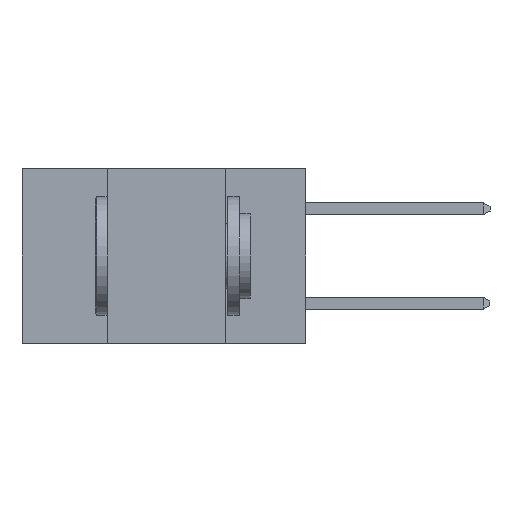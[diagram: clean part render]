
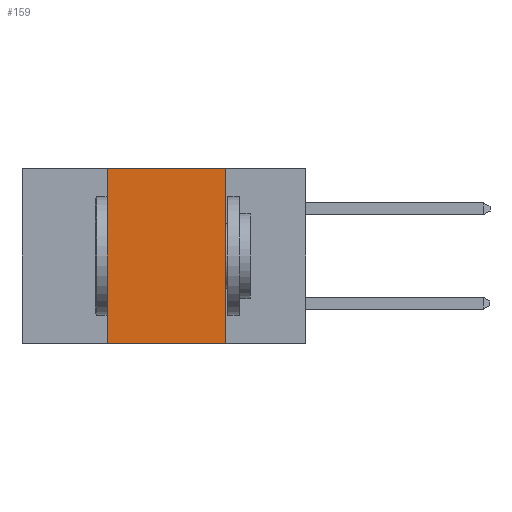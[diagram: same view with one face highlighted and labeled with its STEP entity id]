
A CAD part, left-side view. The second image highlights one B-rep face of the part: STEP entity #159.
In plain terms, the highlighted planar face has unit normal (-1, 0, 0).
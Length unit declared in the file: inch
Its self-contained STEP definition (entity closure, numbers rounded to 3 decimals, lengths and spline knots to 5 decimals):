
#159 = ADVANCED_FACE ( 'NONE', ( #12112 ), #9676, .F. ) ;
#357 = ORIENTED_EDGE ( 'NONE', *, *, #2655, .T. ) ;
#599 = CARTESIAN_POINT ( 'NONE',  ( 0., 0.17, -0.37 ) ) ;
#726 = VECTOR ( 'NONE', #13380, 39.37008 ) ;
#1174 = ORIENTED_EDGE ( 'NONE', *, *, #9477, .F. ) ;
#1383 = CARTESIAN_POINT ( 'NONE',  ( 0., 0.42, 0. ) ) ;
#2437 = DIRECTION ( 'NONE',  ( 0., -1., 0. ) ) ;
#2655 = EDGE_CURVE ( 'NONE', #13415, #5528, #12569, .T. ) ;
#3301 = VERTEX_POINT ( 'NONE', #3535 ) ;
#3443 = EDGE_CURVE ( 'NONE', #13415, #3873, #6007, .T. ) ;
#3535 = CARTESIAN_POINT ( 'NONE',  ( 0., 0.17, 0. ) ) ;
#3538 = LINE ( 'NONE', #6729, #726 ) ;
#3873 = VERTEX_POINT ( 'NONE', #7276 ) ;
#4242 = EDGE_CURVE ( 'NONE', #3301, #5528, #7829, .T. ) ;
#5293 = CARTESIAN_POINT ( 'NONE',  ( 0., 0.17, 0. ) ) ;
#5528 = VERTEX_POINT ( 'NONE', #599 ) ;
#5921 = ORIENTED_EDGE ( 'NONE', *, *, #3443, .F. ) ;
#6007 = LINE ( 'NONE', #1383, #8735 ) ;
#6057 = CARTESIAN_POINT ( 'NONE',  ( 0., 0.6, -0.37 ) ) ;
#6729 = CARTESIAN_POINT ( 'NONE',  ( 0., 0.6, 0. ) ) ;
#6868 = ORIENTED_EDGE ( 'NONE', *, *, #4242, .F. ) ;
#7229 = DIRECTION ( 'NONE',  ( 1., 0., 0. ) ) ;
#7276 = CARTESIAN_POINT ( 'NONE',  ( 0., 0.42, 0. ) ) ;
#7491 = CARTESIAN_POINT ( 'NONE',  ( 0., 0.6, 0. ) ) ;
#7829 = LINE ( 'NONE', #5293, #10468 ) ;
#8735 = VECTOR ( 'NONE', #11108, 39.37008 ) ;
#8996 = CARTESIAN_POINT ( 'NONE',  ( 0., 0.42, -0.37 ) ) ;
#9279 = DIRECTION ( 'NONE',  ( 0., 0., -1. ) ) ;
#9477 = EDGE_CURVE ( 'NONE', #3873, #3301, #3538, .T. ) ;
#9676 = PLANE ( 'NONE',  #14174 ) ;
#10207 = DIRECTION ( 'NONE',  ( 0., 0., -1. ) ) ;
#10468 = VECTOR ( 'NONE', #10207, 39.37008 ) ;
#11108 = DIRECTION ( 'NONE',  ( 0., 0., 1. ) ) ;
#12112 = FACE_OUTER_BOUND ( 'NONE', #12264, .T. ) ;
#12264 = EDGE_LOOP ( 'NONE', ( #6868, #1174, #5921, #357 ) ) ;
#12569 = LINE ( 'NONE', #6057, #12908 ) ;
#12908 = VECTOR ( 'NONE', #2437, 39.37008 ) ;
#13380 = DIRECTION ( 'NONE',  ( 0., -1., 0. ) ) ;
#13415 = VERTEX_POINT ( 'NONE', #8996 ) ;
#14174 = AXIS2_PLACEMENT_3D ( 'NONE', #7491, #7229, #9279 ) ;
